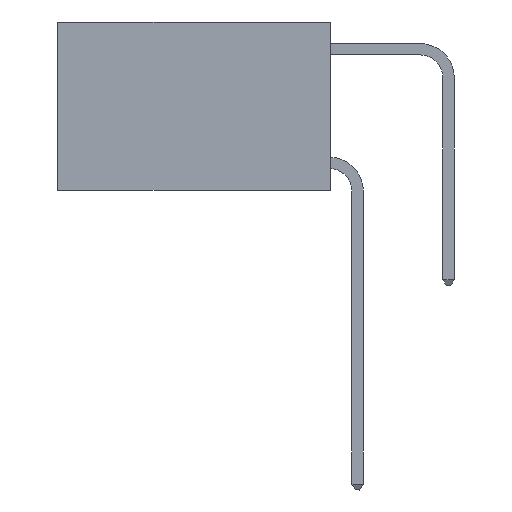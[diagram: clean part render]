
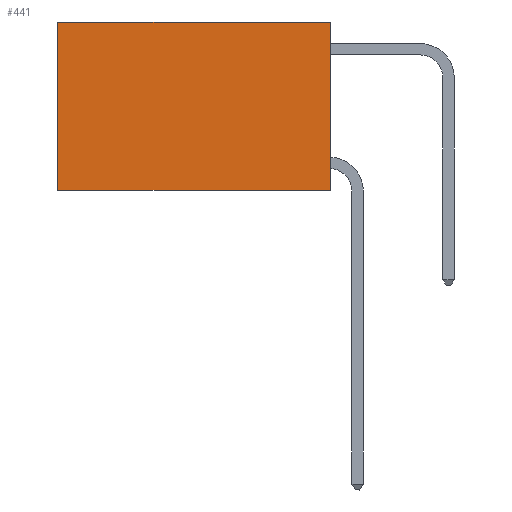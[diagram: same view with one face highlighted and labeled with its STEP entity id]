
A CAD part, left-side view. The second image highlights one B-rep face of the part: STEP entity #441.
In plain terms, the highlighted planar face has unit normal (-1, 0, 0).
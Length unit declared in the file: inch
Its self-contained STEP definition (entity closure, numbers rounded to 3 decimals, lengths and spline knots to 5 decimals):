
#362 = ORIENTED_EDGE ( 'NONE', *, *, #12971, .F. ) ;
#441 = ADVANCED_FACE ( 'NONE', ( #8985 ), #13248, .F. ) ;
#652 = DIRECTION ( 'NONE',  ( 0., 0., -1. ) ) ;
#679 = CARTESIAN_POINT ( 'NONE',  ( 0.2625, 0., -0.37 ) ) ;
#1017 = VERTEX_POINT ( 'NONE', #14632 ) ;
#1434 = DIRECTION ( 'NONE',  ( 0., 1., 0. ) ) ;
#2055 = EDGE_LOOP ( 'NONE', ( #7045, #13750, #362, #12685 ) ) ;
#3220 = EDGE_CURVE ( 'NONE', #11163, #1017, #7372, .T. ) ;
#3966 = VECTOR ( 'NONE', #1434, 39.37008 ) ;
#4734 = CARTESIAN_POINT ( 'NONE',  ( 0.2625, 0.6, -0.37 ) ) ;
#5773 = DIRECTION ( 'NONE',  ( 0., 0., -1. ) ) ;
#6296 = EDGE_CURVE ( 'NONE', #7888, #10860, #7886, .T. ) ;
#6354 = CARTESIAN_POINT ( 'NONE',  ( 0.2625, 0., 0. ) ) ;
#7045 = ORIENTED_EDGE ( 'NONE', *, *, #8668, .T. ) ;
#7372 = LINE ( 'NONE', #8872, #3966 ) ;
#7849 = DIRECTION ( 'NONE',  ( 0., 0., -1. ) ) ;
#7886 = LINE ( 'NONE', #679, #14208 ) ;
#7888 = VERTEX_POINT ( 'NONE', #16398 ) ;
#8445 = CARTESIAN_POINT ( 'NONE',  ( 0.2625, 0.6, 0. ) ) ;
#8668 = EDGE_CURVE ( 'NONE', #1017, #10860, #12684, .T. ) ;
#8872 = CARTESIAN_POINT ( 'NONE',  ( 0.2625, 0., 0. ) ) ;
#8985 = FACE_OUTER_BOUND ( 'NONE', #2055, .T. ) ;
#9327 = VECTOR ( 'NONE', #652, 39.37008 ) ;
#10860 = VERTEX_POINT ( 'NONE', #4734 ) ;
#11163 = VERTEX_POINT ( 'NONE', #15321 ) ;
#12150 = LINE ( 'NONE', #14142, #14963 ) ;
#12684 = LINE ( 'NONE', #8445, #9327 ) ;
#12685 = ORIENTED_EDGE ( 'NONE', *, *, #3220, .T. ) ;
#12971 = EDGE_CURVE ( 'NONE', #11163, #7888, #12150, .T. ) ;
#13248 = PLANE ( 'NONE',  #14646 ) ;
#13750 = ORIENTED_EDGE ( 'NONE', *, *, #6296, .F. ) ;
#14142 = CARTESIAN_POINT ( 'NONE',  ( 0.2625, 0., 0. ) ) ;
#14208 = VECTOR ( 'NONE', #16017, 39.37008 ) ;
#14632 = CARTESIAN_POINT ( 'NONE',  ( 0.2625, 0.6, 0. ) ) ;
#14646 = AXIS2_PLACEMENT_3D ( 'NONE', #6354, #15763, #5773 ) ;
#14963 = VECTOR ( 'NONE', #7849, 39.37008 ) ;
#15321 = CARTESIAN_POINT ( 'NONE',  ( 0.2625, 0., 0. ) ) ;
#15763 = DIRECTION ( 'NONE',  ( 1., 0., 0. ) ) ;
#16017 = DIRECTION ( 'NONE',  ( 0., 1., 0. ) ) ;
#16398 = CARTESIAN_POINT ( 'NONE',  ( 0.2625, 0., -0.37 ) ) ;
